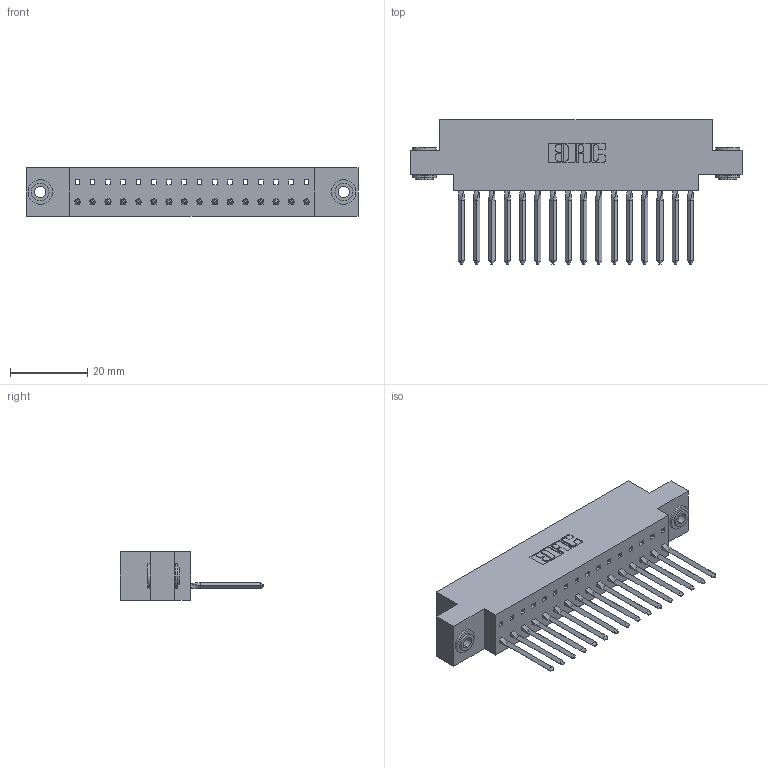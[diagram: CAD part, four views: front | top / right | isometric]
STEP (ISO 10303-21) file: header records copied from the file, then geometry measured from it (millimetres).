
FILE_DESCRIPTION (( 'STEP AP203' ), '1' );
FILE_NAME ('317-016-542-603.STEP', '2020-02-27T15:09:19', ( '' ), ( '' ), 'SwSTEP 2.0', 'SolidWorks 2016', '' );
FILE_SCHEMA (( 'CONFIG_CONTROL_DESIGN' ));
Length unit declared in the file: inch
Products named in the file (4): 317 Part_.156 Dia - TH; 317-016-542-603; 317-290-003_542; 345-250-002_345-250-002-102
Assembly tree (19 placements, depth 2):
  317-016-542-603
    317 Part_.156 Dia - TH
    317-290-003_542  x16
    345-250-002_345-250-002-102  x2
Bounding box: 86.11 x 37.34 x 12.7 mm (x, y, z)
Volume: 12629.1 mm3; surface area: 15044.8 mm2
Topology: 19 solids, 19 shells, 1340 faces, 3823 edges, 2470 vertices
Faces by surface type: plane 1092, cylinder 176, bspline 64, cone 8
Entity records: 25910 total; most frequent: CARTESIAN_POINT 4808, ORIENTED_EDGE 4480, DIRECTION 3822, EDGE_CURVE 2240, LINE 2046, VECTOR 2046, VERTEX_POINT 1486, AXIS2_PLACEMENT_3D 888
